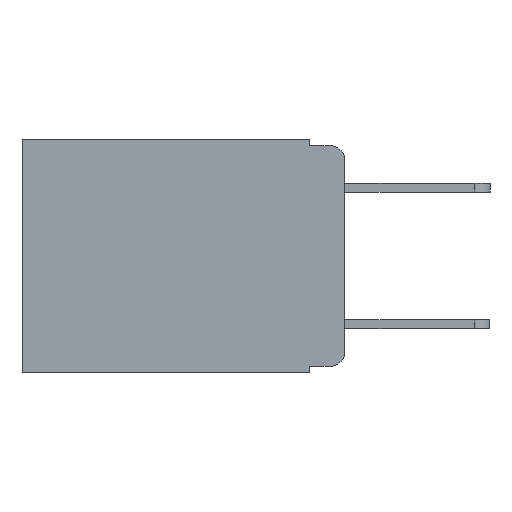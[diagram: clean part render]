
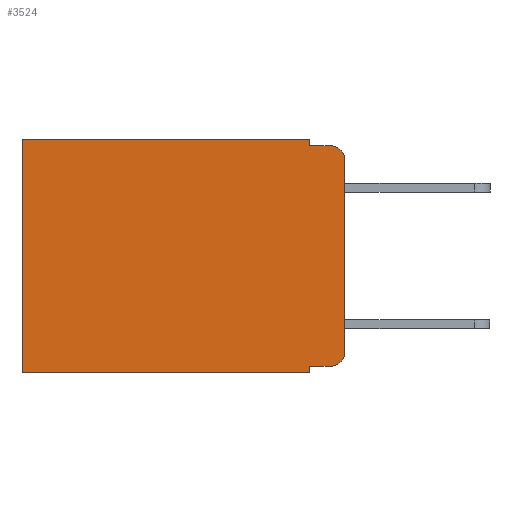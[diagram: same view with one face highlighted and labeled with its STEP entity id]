
A CAD part, left-side view. The second image highlights one B-rep face of the part: STEP entity #3524.
In plain terms, the highlighted planar face has unit normal (-1, 0, 0).
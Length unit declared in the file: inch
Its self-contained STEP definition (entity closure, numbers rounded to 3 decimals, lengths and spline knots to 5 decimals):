
#393 = CARTESIAN_POINT ( 'NONE',  ( 0.298, 0.02, -0.01 ) ) ;
#512 = CARTESIAN_POINT ( 'NONE',  ( 0.298, 0.051, -0.333 ) ) ;
#728 = LINE ( 'NONE', #512, #17339 ) ;
#989 = ORIENTED_EDGE ( 'NONE', *, *, #19611, .F. ) ;
#1374 = DIRECTION ( 'NONE',  ( 0., 0., -1. ) ) ;
#1539 = ORIENTED_EDGE ( 'NONE', *, *, #20730, .F. ) ;
#1777 = VECTOR ( 'NONE', #21202, 39.37008 ) ;
#2802 = DIRECTION ( 'NONE',  ( 0., 0., -1. ) ) ;
#2825 = EDGE_CURVE ( 'NONE', #23726, #19995, #19299, .T. ) ;
#2853 = CARTESIAN_POINT ( 'NONE',  ( 0.298, 0., 0. ) ) ;
#2906 = VERTEX_POINT ( 'NONE', #17927 ) ;
#3029 = FACE_OUTER_BOUND ( 'NONE', #17201, .T. ) ;
#3268 = DIRECTION ( 'NONE',  ( 0., -1., 0. ) ) ;
#3524 = ADVANCED_FACE ( 'NONE', ( #3029 ), #8904, .F. ) ;
#3549 = EDGE_CURVE ( 'NONE', #7661, #2906, #13249, .T. ) ;
#3775 = ORIENTED_EDGE ( 'NONE', *, *, #3549, .T. ) ;
#3830 = LINE ( 'NONE', #20728, #12242 ) ;
#4306 = CARTESIAN_POINT ( 'NONE',  ( 0.298, 0., -0.313 ) ) ;
#4385 = DIRECTION ( 'NONE',  ( 0., -1., 0. ) ) ;
#4858 = VERTEX_POINT ( 'NONE', #20752 ) ;
#5217 = CARTESIAN_POINT ( 'NONE',  ( 0.298, 0.051, -0.01 ) ) ;
#5824 = ORIENTED_EDGE ( 'NONE', *, *, #17621, .T. ) ;
#6569 = CIRCLE ( 'NONE', #7623, 0.02 ) ;
#6910 = LINE ( 'NONE', #19325, #1777 ) ;
#6940 = VECTOR ( 'NONE', #11132, 39.37008 ) ;
#7529 = ORIENTED_EDGE ( 'NONE', *, *, #12550, .F. ) ;
#7553 = DIRECTION ( 'NONE',  ( -1., 0., 0. ) ) ;
#7623 = AXIS2_PLACEMENT_3D ( 'NONE', #19065, #7553, #20941 ) ;
#7661 = VERTEX_POINT ( 'NONE', #19982 ) ;
#7903 = VECTOR ( 'NONE', #3268, 39.37008 ) ;
#7966 = EDGE_CURVE ( 'NONE', #23726, #15284, #3830, .T. ) ;
#8064 = ORIENTED_EDGE ( 'NONE', *, *, #2825, .T. ) ;
#8493 = LINE ( 'NONE', #5217, #7903 ) ;
#8885 = CARTESIAN_POINT ( 'NONE',  ( 0.298, 0.473, -0.343 ) ) ;
#8904 = PLANE ( 'NONE',  #23419 ) ;
#8989 = CARTESIAN_POINT ( 'NONE',  ( 0.298, 0., 0. ) ) ;
#9574 = DIRECTION ( 'NONE',  ( 0., 0., -1. ) ) ;
#10407 = VECTOR ( 'NONE', #9574, 39.37008 ) ;
#10731 = CARTESIAN_POINT ( 'NONE',  ( 0.298, 0.02, -0.03 ) ) ;
#10739 = ORIENTED_EDGE ( 'NONE', *, *, #18068, .T. ) ;
#11016 = DIRECTION ( 'NONE',  ( -1., 0., 0. ) ) ;
#11023 = LINE ( 'NONE', #22831, #10407 ) ;
#11132 = DIRECTION ( 'NONE',  ( 0., 1., 0. ) ) ;
#11650 = AXIS2_PLACEMENT_3D ( 'NONE', #10731, #11016, #22698 ) ;
#11906 = CARTESIAN_POINT ( 'NONE',  ( 0.298, 0., -0.03 ) ) ;
#12242 = VECTOR ( 'NONE', #22612, 39.37008 ) ;
#12428 = CARTESIAN_POINT ( 'NONE',  ( 0.298, 0.051, -0.01 ) ) ;
#12525 = CARTESIAN_POINT ( 'NONE',  ( 0.298, 0.051, -0.343 ) ) ;
#12550 = EDGE_CURVE ( 'NONE', #7661, #15498, #21316, .T. ) ;
#12850 = CARTESIAN_POINT ( 'NONE',  ( 0.298, 0.051, 0. ) ) ;
#13249 = LINE ( 'NONE', #2853, #6940 ) ;
#13308 = DIRECTION ( 'NONE',  ( 0., 0., -1. ) ) ;
#13341 = DIRECTION ( 'NONE',  ( 1., 0., 0. ) ) ;
#13926 = EDGE_CURVE ( 'NONE', #4858, #15284, #6569, .T. ) ;
#14116 = VERTEX_POINT ( 'NONE', #15878 ) ;
#14318 = CARTESIAN_POINT ( 'NONE',  ( 0.298, 0.051, 0. ) ) ;
#14965 = ORIENTED_EDGE ( 'NONE', *, *, #21154, .F. ) ;
#15284 = VERTEX_POINT ( 'NONE', #4306 ) ;
#15498 = VERTEX_POINT ( 'NONE', #12428 ) ;
#15733 = ORIENTED_EDGE ( 'NONE', *, *, #7966, .F. ) ;
#15878 = CARTESIAN_POINT ( 'NONE',  ( 0.298, 0.051, -0.333 ) ) ;
#16277 = VECTOR ( 'NONE', #1374, 39.37008 ) ;
#17158 = VECTOR ( 'NONE', #2802, 39.37008 ) ;
#17201 = EDGE_LOOP ( 'NONE', ( #15733, #8064, #989, #7529, #3775, #10739, #14965, #1539, #5824, #19112 ) ) ;
#17339 = VECTOR ( 'NONE', #4385, 39.37008 ) ;
#17621 = EDGE_CURVE ( 'NONE', #14116, #4858, #728, .T. ) ;
#17927 = CARTESIAN_POINT ( 'NONE',  ( 0.298, 0.473, 0. ) ) ;
#18068 = EDGE_CURVE ( 'NONE', #2906, #18468, #11023, .T. ) ;
#18468 = VERTEX_POINT ( 'NONE', #8885 ) ;
#19065 = CARTESIAN_POINT ( 'NONE',  ( 0.298, 0.02, -0.313 ) ) ;
#19112 = ORIENTED_EDGE ( 'NONE', *, *, #13926, .T. ) ;
#19299 = CIRCLE ( 'NONE', #11650, 0.02 ) ;
#19325 = CARTESIAN_POINT ( 'NONE',  ( 0.298, 0., -0.343 ) ) ;
#19611 = EDGE_CURVE ( 'NONE', #15498, #19995, #8493, .T. ) ;
#19982 = CARTESIAN_POINT ( 'NONE',  ( 0.298, 0.051, 0. ) ) ;
#19995 = VERTEX_POINT ( 'NONE', #393 ) ;
#20728 = CARTESIAN_POINT ( 'NONE',  ( 0.298, 0., 0. ) ) ;
#20730 = EDGE_CURVE ( 'NONE', #14116, #20802, #22174, .T. ) ;
#20752 = CARTESIAN_POINT ( 'NONE',  ( 0.298, 0.02, -0.333 ) ) ;
#20802 = VERTEX_POINT ( 'NONE', #12525 ) ;
#20941 = DIRECTION ( 'NONE',  ( 0., 0., -1. ) ) ;
#21154 = EDGE_CURVE ( 'NONE', #20802, #18468, #6910, .T. ) ;
#21202 = DIRECTION ( 'NONE',  ( 0., 1., 0. ) ) ;
#21316 = LINE ( 'NONE', #12850, #16277 ) ;
#22174 = LINE ( 'NONE', #14318, #17158 ) ;
#22612 = DIRECTION ( 'NONE',  ( 0., 0., -1. ) ) ;
#22698 = DIRECTION ( 'NONE',  ( 0., 0., -1. ) ) ;
#22831 = CARTESIAN_POINT ( 'NONE',  ( 0.298, 0.473, 0. ) ) ;
#23419 = AXIS2_PLACEMENT_3D ( 'NONE', #8989, #13341, #13308 ) ;
#23726 = VERTEX_POINT ( 'NONE', #11906 ) ;
